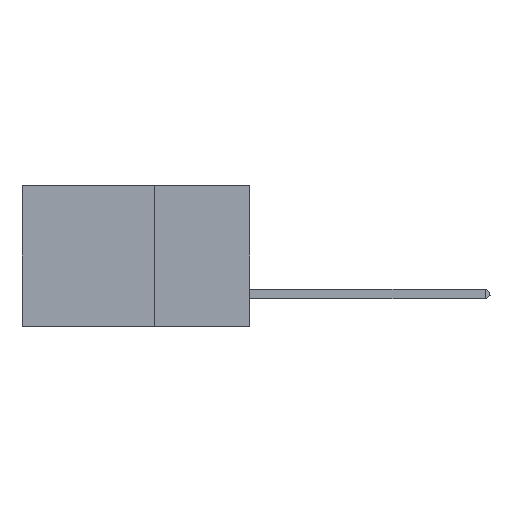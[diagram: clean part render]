
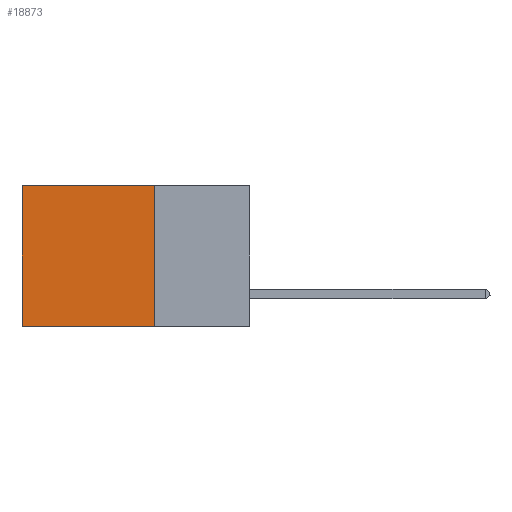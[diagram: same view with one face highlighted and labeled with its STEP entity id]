
A CAD part, left-side view. The second image highlights one B-rep face of the part: STEP entity #18873.
In plain terms, the highlighted planar face has unit normal (-1, 0, 0).
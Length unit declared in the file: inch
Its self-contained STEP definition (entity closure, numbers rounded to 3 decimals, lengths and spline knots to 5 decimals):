
#1753 = CARTESIAN_POINT ( 'NONE',  ( 0.2875, 0.6, 0. ) ) ;
#2043 = CARTESIAN_POINT ( 'NONE',  ( 0.2875, 0.25, 0. ) ) ;
#2474 = VERTEX_POINT ( 'NONE', #20029 ) ;
#2677 = ORIENTED_EDGE ( 'NONE', *, *, #3433, .F. ) ;
#2678 = DIRECTION ( 'NONE',  ( 0., 0., -1. ) ) ;
#2894 = CARTESIAN_POINT ( 'NONE',  ( 0.2875, 0.6, 0. ) ) ;
#3433 = EDGE_CURVE ( 'NONE', #2474, #29297, #12205, .T. ) ;
#6501 = DIRECTION ( 'NONE',  ( 1., 0., 0. ) ) ;
#7769 = VERTEX_POINT ( 'NONE', #2043 ) ;
#9715 = DIRECTION ( 'NONE',  ( 0., 1., 0. ) ) ;
#11221 = VECTOR ( 'NONE', #19627, 39.37008 ) ;
#11920 = DIRECTION ( 'NONE',  ( 0., 1., 0. ) ) ;
#12039 = VECTOR ( 'NONE', #23793, 39.37008 ) ;
#12205 = LINE ( 'NONE', #25364, #27152 ) ;
#13148 = PLANE ( 'NONE',  #32943 ) ;
#13503 = CARTESIAN_POINT ( 'NONE',  ( 0.2875, 0.25, 0. ) ) ;
#14403 = LINE ( 'NONE', #19847, #29877 ) ;
#16868 = FACE_OUTER_BOUND ( 'NONE', #26802, .T. ) ;
#18873 = ADVANCED_FACE ( 'NONE', ( #16868 ), #13148, .F. ) ;
#19627 = DIRECTION ( 'NONE',  ( 0., 0., -1. ) ) ;
#19847 = CARTESIAN_POINT ( 'NONE',  ( 0.2875, 0.25, 0. ) ) ;
#20029 = CARTESIAN_POINT ( 'NONE',  ( 0.2875, 0.25, -0.37 ) ) ;
#20579 = ORIENTED_EDGE ( 'NONE', *, *, #36225, .F. ) ;
#20777 = LINE ( 'NONE', #13503, #12039 ) ;
#23457 = CARTESIAN_POINT ( 'NONE',  ( 0.2875, 0.25, 0. ) ) ;
#23793 = DIRECTION ( 'NONE',  ( 0., 0., -1. ) ) ;
#25364 = CARTESIAN_POINT ( 'NONE',  ( 0.2875, 0.25, -0.37 ) ) ;
#26226 = ORIENTED_EDGE ( 'NONE', *, *, #28920, .T. ) ;
#26802 = EDGE_LOOP ( 'NONE', ( #26226, #2677, #20579, #43743 ) ) ;
#27152 = VECTOR ( 'NONE', #11920, 39.37008 ) ;
#28920 = EDGE_CURVE ( 'NONE', #40490, #29297, #43674, .T. ) ;
#29297 = VERTEX_POINT ( 'NONE', #34501 ) ;
#29877 = VECTOR ( 'NONE', #9715, 39.37008 ) ;
#32943 = AXIS2_PLACEMENT_3D ( 'NONE', #23457, #6501, #2678 ) ;
#34501 = CARTESIAN_POINT ( 'NONE',  ( 0.2875, 0.6, -0.37 ) ) ;
#36225 = EDGE_CURVE ( 'NONE', #7769, #2474, #20777, .T. ) ;
#40490 = VERTEX_POINT ( 'NONE', #1753 ) ;
#40691 = EDGE_CURVE ( 'NONE', #7769, #40490, #14403, .T. ) ;
#43674 = LINE ( 'NONE', #2894, #11221 ) ;
#43743 = ORIENTED_EDGE ( 'NONE', *, *, #40691, .T. ) ;
